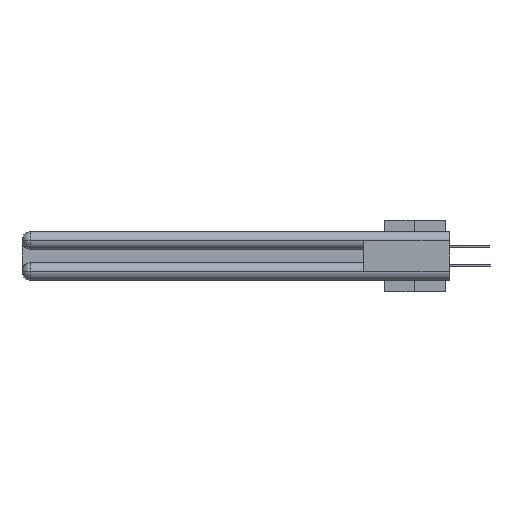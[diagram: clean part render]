
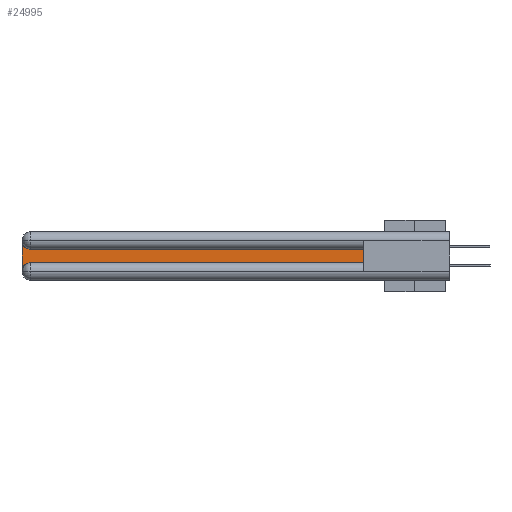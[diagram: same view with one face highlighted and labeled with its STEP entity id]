
A CAD part, left-side view. The second image highlights one B-rep face of the part: STEP entity #24995.
In plain terms, the highlighted planar face has unit normal (-1, 0, 0).
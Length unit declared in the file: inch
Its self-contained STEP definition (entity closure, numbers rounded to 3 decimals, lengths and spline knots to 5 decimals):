
#249 = ORIENTED_EDGE ( 'NONE', *, *, #19483, .T. ) ;
#754 = DIRECTION ( 'NONE',  ( 0., 0., -1. ) ) ;
#922 = EDGE_CURVE ( 'NONE', #6881, #32192, #19293, .T. ) ;
#1048 = VECTOR ( 'NONE', #24293, 39.37008 ) ;
#1272 = DIRECTION ( 'NONE',  ( 0., 0., -1. ) ) ;
#2354 = CARTESIAN_POINT ( 'NONE',  ( 0.075, 2.94, -0.0625 ) ) ;
#2868 = AXIS2_PLACEMENT_3D ( 'NONE', #6732, #29357, #6852 ) ;
#3264 = CARTESIAN_POINT ( 'NONE',  ( 0.075, 3., -0.2775 ) ) ;
#4279 = VECTOR ( 'NONE', #25035, 39.37008 ) ;
#4543 = EDGE_LOOP ( 'NONE', ( #32119, #14925, #19304, #249, #16017, #24139 ) ) ;
#4643 = AXIS2_PLACEMENT_3D ( 'NONE', #9619, #10099, #1272 ) ;
#5007 = CARTESIAN_POINT ( 'NONE',  ( 0.075, 2.94, -0.1225 ) ) ;
#5289 = DIRECTION ( 'NONE',  ( 1., 0., 0. ) ) ;
#5663 = EDGE_CURVE ( 'NONE', #32192, #12923, #24783, .T. ) ;
#6560 = VERTEX_POINT ( 'NONE', #33996 ) ;
#6732 = CARTESIAN_POINT ( 'NONE',  ( 0.075, 3., -0.1225 ) ) ;
#6768 = AXIS2_PLACEMENT_3D ( 'NONE', #2354, #5289, #13447 ) ;
#6852 = DIRECTION ( 'NONE',  ( 0., 0., -1. ) ) ;
#6881 = VERTEX_POINT ( 'NONE', #33105 ) ;
#7915 = FACE_OUTER_BOUND ( 'NONE', #4543, .T. ) ;
#9246 = CIRCLE ( 'NONE', #4643, 0.06 ) ;
#9619 = CARTESIAN_POINT ( 'NONE',  ( 0.075, 2.94, -0.2775 ) ) ;
#9677 = PLANE ( 'NONE',  #2868 ) ;
#10099 = DIRECTION ( 'NONE',  ( 1., 0., 0. ) ) ;
#12504 = EDGE_CURVE ( 'NONE', #12923, #31509, #33476, .T. ) ;
#12923 = VERTEX_POINT ( 'NONE', #5007 ) ;
#13447 = DIRECTION ( 'NONE',  ( 0., 0., -1. ) ) ;
#14021 = LINE ( 'NONE', #23209, #33942 ) ;
#14910 = VERTEX_POINT ( 'NONE', #3264 ) ;
#14925 = ORIENTED_EDGE ( 'NONE', *, *, #12504, .T. ) ;
#16017 = ORIENTED_EDGE ( 'NONE', *, *, #32462, .T. ) ;
#17139 = DIRECTION ( 'NONE',  ( 0., 1., 0. ) ) ;
#19293 = LINE ( 'NONE', #24903, #4279 ) ;
#19304 = ORIENTED_EDGE ( 'NONE', *, *, #26796, .T. ) ;
#19483 = EDGE_CURVE ( 'NONE', #14910, #6560, #9246, .T. ) ;
#21944 = CARTESIAN_POINT ( 'NONE',  ( 0.075, 3., -0.0625 ) ) ;
#22197 = LINE ( 'NONE', #26791, #1048 ) ;
#23209 = CARTESIAN_POINT ( 'NONE',  ( 0.075, 3., -0.2175 ) ) ;
#24139 = ORIENTED_EDGE ( 'NONE', *, *, #922, .T. ) ;
#24293 = DIRECTION ( 'NONE',  ( 0., -1., 0. ) ) ;
#24783 = LINE ( 'NONE', #28505, #33245 ) ;
#24895 = CARTESIAN_POINT ( 'NONE',  ( 0.075, 0.6, -0.1225 ) ) ;
#24903 = CARTESIAN_POINT ( 'NONE',  ( 0.075, 0.6, -0.2175 ) ) ;
#24995 = ADVANCED_FACE ( 'NONE', ( #7915 ), #9677, .F. ) ;
#25035 = DIRECTION ( 'NONE',  ( 0., 0., 1. ) ) ;
#26791 = CARTESIAN_POINT ( 'NONE',  ( 0.075, 0.6, -0.2175 ) ) ;
#26796 = EDGE_CURVE ( 'NONE', #31509, #14910, #14021, .T. ) ;
#28505 = CARTESIAN_POINT ( 'NONE',  ( 0.075, 0.6, -0.1225 ) ) ;
#29357 = DIRECTION ( 'NONE',  ( 1., 0., 0. ) ) ;
#31509 = VERTEX_POINT ( 'NONE', #21944 ) ;
#32119 = ORIENTED_EDGE ( 'NONE', *, *, #5663, .T. ) ;
#32192 = VERTEX_POINT ( 'NONE', #24895 ) ;
#32462 = EDGE_CURVE ( 'NONE', #6560, #6881, #22197, .T. ) ;
#33105 = CARTESIAN_POINT ( 'NONE',  ( 0.075, 0.6, -0.2175 ) ) ;
#33245 = VECTOR ( 'NONE', #17139, 39.37008 ) ;
#33476 = CIRCLE ( 'NONE', #6768, 0.06 ) ;
#33942 = VECTOR ( 'NONE', #754, 39.37008 ) ;
#33996 = CARTESIAN_POINT ( 'NONE',  ( 0.075, 2.94, -0.2175 ) ) ;
